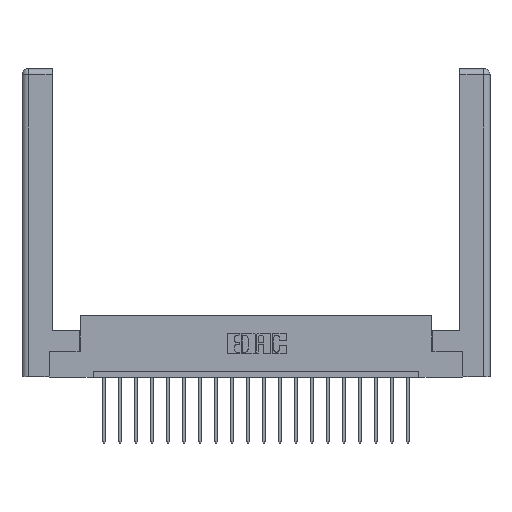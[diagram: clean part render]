
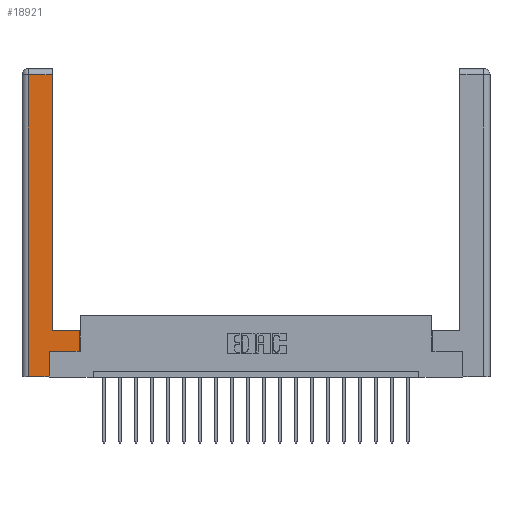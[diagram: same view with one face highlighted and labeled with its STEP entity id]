
A CAD part, top view. The second image highlights one B-rep face of the part: STEP entity #18921.
In plain terms, the highlighted planar face has unit normal (0, 0, 1).
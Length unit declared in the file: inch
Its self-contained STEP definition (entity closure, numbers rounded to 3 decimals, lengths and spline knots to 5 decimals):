
#587 = CARTESIAN_POINT ( 'NONE',  ( 0.265, 0., 0. ) ) ;
#896 = ORIENTED_EDGE ( 'NONE', *, *, #9933, .T. ) ;
#937 = LINE ( 'NONE', #2094, #15260 ) ;
#1068 = CARTESIAN_POINT ( 'NONE',  ( 0.0615, 0., 0. ) ) ;
#1152 = CARTESIAN_POINT ( 'NONE',  ( 0.265, 0., 0. ) ) ;
#1194 = EDGE_CURVE ( 'NONE', #13718, #12776, #9572, .T. ) ;
#1284 = DIRECTION ( 'NONE',  ( -1., 0., 0. ) ) ;
#1560 = VERTEX_POINT ( 'NONE', #3595 ) ;
#2094 = CARTESIAN_POINT ( 'NONE',  ( 0.565, 0.45, 0. ) ) ;
#2399 = CARTESIAN_POINT ( 'NONE',  ( 0.265, 0.245, 0. ) ) ;
#2554 = CARTESIAN_POINT ( 'NONE',  ( 0.295, 3., 0. ) ) ;
#2813 = EDGE_CURVE ( 'NONE', #17426, #19695, #12229, .T. ) ;
#2976 = AXIS2_PLACEMENT_3D ( 'NONE', #14094, #9603, #20321 ) ;
#3595 = CARTESIAN_POINT ( 'NONE',  ( 0.565, 0.245, 0. ) ) ;
#3633 = ORIENTED_EDGE ( 'NONE', *, *, #7460, .T. ) ;
#4133 = DIRECTION ( 'NONE',  ( 0., 1., 0. ) ) ;
#4791 = VECTOR ( 'NONE', #11298, 39.37008 ) ;
#5330 = ORIENTED_EDGE ( 'NONE', *, *, #2813, .T. ) ;
#5557 = VERTEX_POINT ( 'NONE', #13899 ) ;
#5653 = CARTESIAN_POINT ( 'NONE',  ( 0.295, 0.45, 0. ) ) ;
#5862 = VERTEX_POINT ( 'NONE', #14759 ) ;
#6490 = EDGE_CURVE ( 'NONE', #18188, #1560, #12602, .T. ) ;
#6650 = VECTOR ( 'NONE', #1284, 39.37008 ) ;
#6704 = DIRECTION ( 'NONE',  ( 0., 1., 0. ) ) ;
#7460 = EDGE_CURVE ( 'NONE', #5862, #17426, #11064, .T. ) ;
#8070 = CARTESIAN_POINT ( 'NONE',  ( 0.565, 0.245, 0. ) ) ;
#8541 = VECTOR ( 'NONE', #4133, 39.37008 ) ;
#8581 = ORIENTED_EDGE ( 'NONE', *, *, #18636, .T. ) ;
#8714 = FACE_OUTER_BOUND ( 'NONE', #9835, .T. ) ;
#8733 = VECTOR ( 'NONE', #16302, 39.37008 ) ;
#9572 = LINE ( 'NONE', #587, #12037 ) ;
#9603 = DIRECTION ( 'NONE',  ( 0., 0., -1. ) ) ;
#9625 = DIRECTION ( 'NONE',  ( 1., 0., 0. ) ) ;
#9721 = CARTESIAN_POINT ( 'NONE',  ( 0.0615, 2.94, 0. ) ) ;
#9835 = EDGE_LOOP ( 'NONE', ( #5330, #16293, #896, #14653, #8581, #10765, #13255, #3633 ) ) ;
#9933 = EDGE_CURVE ( 'NONE', #5557, #13718, #17627, .T. ) ;
#10107 = DIRECTION ( 'NONE',  ( 1., 0., 0. ) ) ;
#10765 = ORIENTED_EDGE ( 'NONE', *, *, #6490, .T. ) ;
#10920 = EDGE_CURVE ( 'NONE', #19695, #5557, #13171, .T. ) ;
#11064 = LINE ( 'NONE', #13500, #6650 ) ;
#11103 = CARTESIAN_POINT ( 'NONE',  ( 0.295, 2.94, 0. ) ) ;
#11298 = DIRECTION ( 'NONE',  ( -1., 0., 0. ) ) ;
#12037 = VECTOR ( 'NONE', #10107, 39.37008 ) ;
#12229 = LINE ( 'NONE', #2554, #8541 ) ;
#12602 = LINE ( 'NONE', #8070, #17730 ) ;
#12709 = PLANE ( 'NONE',  #2976 ) ;
#12776 = VERTEX_POINT ( 'NONE', #1152 ) ;
#13171 = LINE ( 'NONE', #9721, #4791 ) ;
#13255 = ORIENTED_EDGE ( 'NONE', *, *, #15720, .T. ) ;
#13500 = CARTESIAN_POINT ( 'NONE',  ( 0.295, 0.45, 0. ) ) ;
#13630 = DIRECTION ( 'NONE',  ( 0., -1., 0. ) ) ;
#13718 = VERTEX_POINT ( 'NONE', #19215 ) ;
#13899 = CARTESIAN_POINT ( 'NONE',  ( 0.0615, 2.94, 0. ) ) ;
#14094 = CARTESIAN_POINT ( 'NONE',  ( 0., 0., 0. ) ) ;
#14653 = ORIENTED_EDGE ( 'NONE', *, *, #1194, .T. ) ;
#14759 = CARTESIAN_POINT ( 'NONE',  ( 0.565, 0.45, 0. ) ) ;
#15260 = VECTOR ( 'NONE', #6704, 39.37008 ) ;
#15388 = LINE ( 'NONE', #16385, #8733 ) ;
#15720 = EDGE_CURVE ( 'NONE', #1560, #5862, #937, .T. ) ;
#16293 = ORIENTED_EDGE ( 'NONE', *, *, #10920, .T. ) ;
#16302 = DIRECTION ( 'NONE',  ( 0., 1., 0. ) ) ;
#16385 = CARTESIAN_POINT ( 'NONE',  ( 0.265, 0.245, 0. ) ) ;
#16661 = VECTOR ( 'NONE', #13630, 39.37008 ) ;
#17426 = VERTEX_POINT ( 'NONE', #5653 ) ;
#17627 = LINE ( 'NONE', #1068, #16661 ) ;
#17730 = VECTOR ( 'NONE', #9625, 39.37008 ) ;
#18188 = VERTEX_POINT ( 'NONE', #2399 ) ;
#18636 = EDGE_CURVE ( 'NONE', #12776, #18188, #15388, .T. ) ;
#18921 = ADVANCED_FACE ( 'NONE', ( #8714 ), #12709, .F. ) ;
#19215 = CARTESIAN_POINT ( 'NONE',  ( 0.0615, 0., 0. ) ) ;
#19695 = VERTEX_POINT ( 'NONE', #11103 ) ;
#20321 = DIRECTION ( 'NONE',  ( -1., 0., 0. ) ) ;
